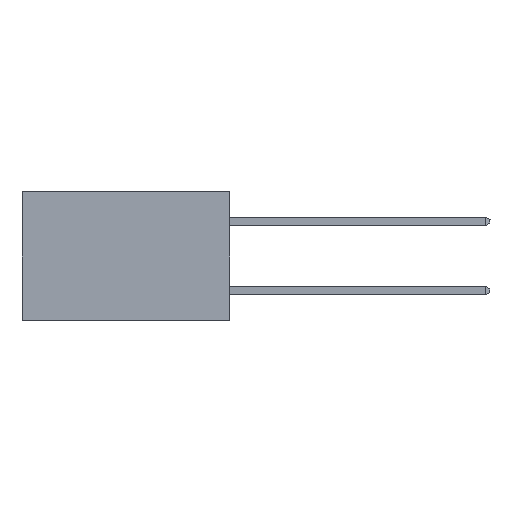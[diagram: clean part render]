
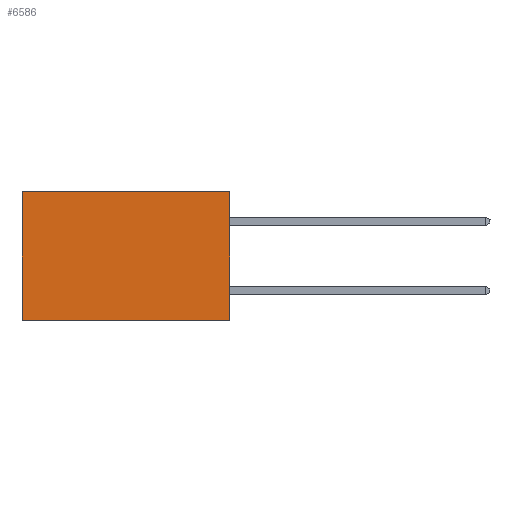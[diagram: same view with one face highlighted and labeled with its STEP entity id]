
A CAD part, left-side view. The second image highlights one B-rep face of the part: STEP entity #6586.
In plain terms, the highlighted planar face has unit normal (-1, 0, 0).
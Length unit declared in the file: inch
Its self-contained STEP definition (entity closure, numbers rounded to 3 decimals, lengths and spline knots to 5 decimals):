
#453 = DIRECTION ( 'NONE',  ( 0., 1., 0. ) ) ;
#1522 = DIRECTION ( 'NONE',  ( 0., 0., -1. ) ) ;
#1604 = FACE_OUTER_BOUND ( 'NONE', #3394, .T. ) ;
#1647 = EDGE_CURVE ( 'NONE', #3077, #6313, #15348, .T. ) ;
#1820 = EDGE_CURVE ( 'NONE', #6313, #2528, #14942, .T. ) ;
#2264 = ORIENTED_EDGE ( 'NONE', *, *, #9493, .T. ) ;
#2528 = VERTEX_POINT ( 'NONE', #14114 ) ;
#2664 = ORIENTED_EDGE ( 'NONE', *, *, #9424, .T. ) ;
#3077 = VERTEX_POINT ( 'NONE', #11971 ) ;
#3394 = EDGE_LOOP ( 'NONE', ( #2664, #11922, #15338, #2264 ) ) ;
#4272 = VECTOR ( 'NONE', #7229, 39.37008 ) ;
#4860 = VECTOR ( 'NONE', #453, 39.37008 ) ;
#6287 = AXIS2_PLACEMENT_3D ( 'NONE', #14535, #7225, #1522 ) ;
#6313 = VERTEX_POINT ( 'NONE', #11410 ) ;
#6356 = VECTOR ( 'NONE', #13377, 39.37008 ) ;
#6586 = ADVANCED_FACE ( 'NONE', ( #1604 ), #8802, .F. ) ;
#7225 = DIRECTION ( 'NONE',  ( 1., 0., 0. ) ) ;
#7229 = DIRECTION ( 'NONE',  ( 0., 0., -1. ) ) ;
#7415 = LINE ( 'NONE', #10079, #6356 ) ;
#7694 = CARTESIAN_POINT ( 'NONE',  ( 0.2615, 0.6, 0. ) ) ;
#8802 = PLANE ( 'NONE',  #6287 ) ;
#9424 = EDGE_CURVE ( 'NONE', #13240, #2528, #10872, .T. ) ;
#9493 = EDGE_CURVE ( 'NONE', #3077, #13240, #7415, .T. ) ;
#10079 = CARTESIAN_POINT ( 'NONE',  ( 0.2615, 0., 0. ) ) ;
#10872 = LINE ( 'NONE', #10952, #15377 ) ;
#10952 = CARTESIAN_POINT ( 'NONE',  ( 0.2615, 0.6, -0.37 ) ) ;
#11410 = CARTESIAN_POINT ( 'NONE',  ( 0.2615, 0., -0.37 ) ) ;
#11922 = ORIENTED_EDGE ( 'NONE', *, *, #1820, .F. ) ;
#11971 = CARTESIAN_POINT ( 'NONE',  ( 0.2615, 0., 0. ) ) ;
#12275 = CARTESIAN_POINT ( 'NONE',  ( 0.2615, 0., -0.37 ) ) ;
#13240 = VERTEX_POINT ( 'NONE', #7694 ) ;
#13377 = DIRECTION ( 'NONE',  ( 0., 1., 0. ) ) ;
#14114 = CARTESIAN_POINT ( 'NONE',  ( 0.2615, 0.6, -0.37 ) ) ;
#14470 = CARTESIAN_POINT ( 'NONE',  ( 0.2615, 0., -0.37 ) ) ;
#14480 = DIRECTION ( 'NONE',  ( 0., 0., -1. ) ) ;
#14535 = CARTESIAN_POINT ( 'NONE',  ( 0.2615, 0., -0.37 ) ) ;
#14942 = LINE ( 'NONE', #12275, #4860 ) ;
#15338 = ORIENTED_EDGE ( 'NONE', *, *, #1647, .F. ) ;
#15348 = LINE ( 'NONE', #14470, #4272 ) ;
#15377 = VECTOR ( 'NONE', #14480, 39.37008 ) ;
